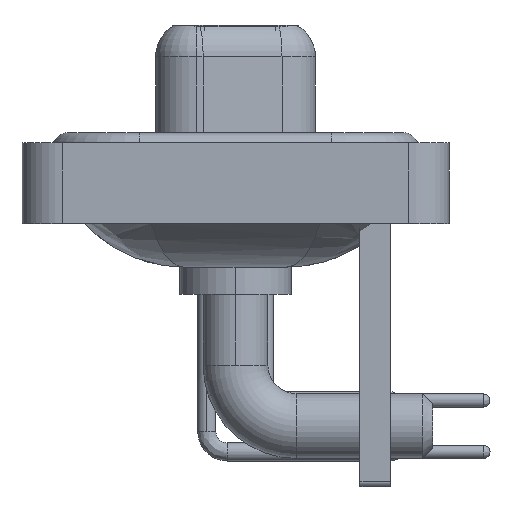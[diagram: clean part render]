
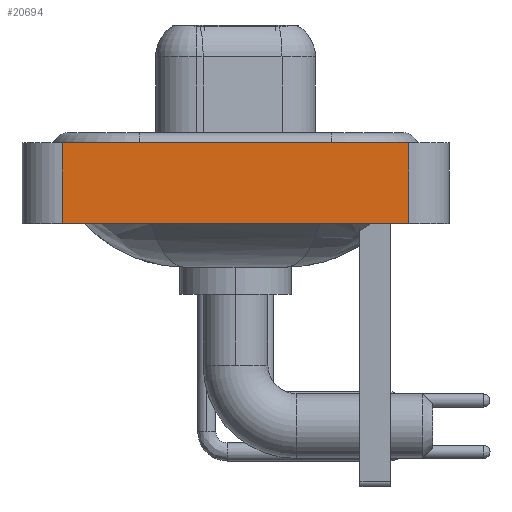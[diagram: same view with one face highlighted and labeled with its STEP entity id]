
A CAD part, left-side view. The second image highlights one B-rep face of the part: STEP entity #20694.
In plain terms, the highlighted planar face has unit normal (-1, 0, 0).
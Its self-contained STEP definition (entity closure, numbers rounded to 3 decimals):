
#2330 = VECTOR ( 'NONE', #6030, 1000. ) ;
#3305 = ORIENTED_EDGE ( 'NONE', *, *, #10364, .T. ) ;
#3692 = EDGE_CURVE ( 'NONE', #5497, #20421, #14543, .T. ) ;
#3920 = VECTOR ( 'NONE', #5909, 1000. ) ;
#5129 = VECTOR ( 'NONE', #12656, 1000. ) ;
#5419 = EDGE_LOOP ( 'NONE', ( #3305, #12493, #19486, #16604 ) ) ;
#5497 = VERTEX_POINT ( 'NONE', #14301 ) ;
#5805 = LINE ( 'NONE', #17871, #3920 ) ;
#5909 = DIRECTION ( 'NONE',  ( 0., -1., 0. ) ) ;
#6024 = CARTESIAN_POINT ( 'NONE',  ( -7.35, -8.55, -3.6 ) ) ;
#6030 = DIRECTION ( 'NONE',  ( 0., 0., 1. ) ) ;
#7072 = EDGE_CURVE ( 'NONE', #16157, #14735, #5805, .T. ) ;
#7682 = DIRECTION ( 'NONE',  ( 0., 0., 1. ) ) ;
#8152 = AXIS2_PLACEMENT_3D ( 'NONE', #9127, #19200, #7682 ) ;
#9127 = CARTESIAN_POINT ( 'NONE',  ( -7.35, -8.55, -3.6 ) ) ;
#9307 = CARTESIAN_POINT ( 'NONE',  ( -7.35, -8.55, 0.4 ) ) ;
#9444 = EDGE_CURVE ( 'NONE', #5497, #16157, #13080, .T. ) ;
#9878 = DIRECTION ( 'NONE',  ( 0., 0., 1. ) ) ;
#10364 = EDGE_CURVE ( 'NONE', #20421, #14735, #20183, .T. ) ;
#11190 = VECTOR ( 'NONE', #9878, 1000. ) ;
#12493 = ORIENTED_EDGE ( 'NONE', *, *, #7072, .F. ) ;
#12656 = DIRECTION ( 'NONE',  ( 0., -1., 0. ) ) ;
#12980 = CARTESIAN_POINT ( 'NONE',  ( -7.35, 8.55, -3.6 ) ) ;
#13080 = LINE ( 'NONE', #12980, #2330 ) ;
#13527 = CARTESIAN_POINT ( 'NONE',  ( -7.35, -8.55, -3.6 ) ) ;
#14301 = CARTESIAN_POINT ( 'NONE',  ( -7.35, 8.55, -3.6 ) ) ;
#14543 = LINE ( 'NONE', #6024, #5129 ) ;
#14660 = CARTESIAN_POINT ( 'NONE',  ( -7.35, -8.55, -3.6 ) ) ;
#14735 = VERTEX_POINT ( 'NONE', #9307 ) ;
#15021 = CARTESIAN_POINT ( 'NONE',  ( -7.35, 8.55, 0.4 ) ) ;
#16157 = VERTEX_POINT ( 'NONE', #15021 ) ;
#16604 = ORIENTED_EDGE ( 'NONE', *, *, #3692, .T. ) ;
#17871 = CARTESIAN_POINT ( 'NONE',  ( -7.35, -8.55, 0.4 ) ) ;
#19200 = DIRECTION ( 'NONE',  ( -1., 0., 0. ) ) ;
#19486 = ORIENTED_EDGE ( 'NONE', *, *, #9444, .F. ) ;
#20183 = LINE ( 'NONE', #13527, #11190 ) ;
#20205 = FACE_OUTER_BOUND ( 'NONE', #5419, .T. ) ;
#20421 = VERTEX_POINT ( 'NONE', #14660 ) ;
#20694 = ADVANCED_FACE ( 'NONE', ( #20205 ), #20993, .T. ) ;
#20993 = PLANE ( 'NONE',  #8152 ) ;
